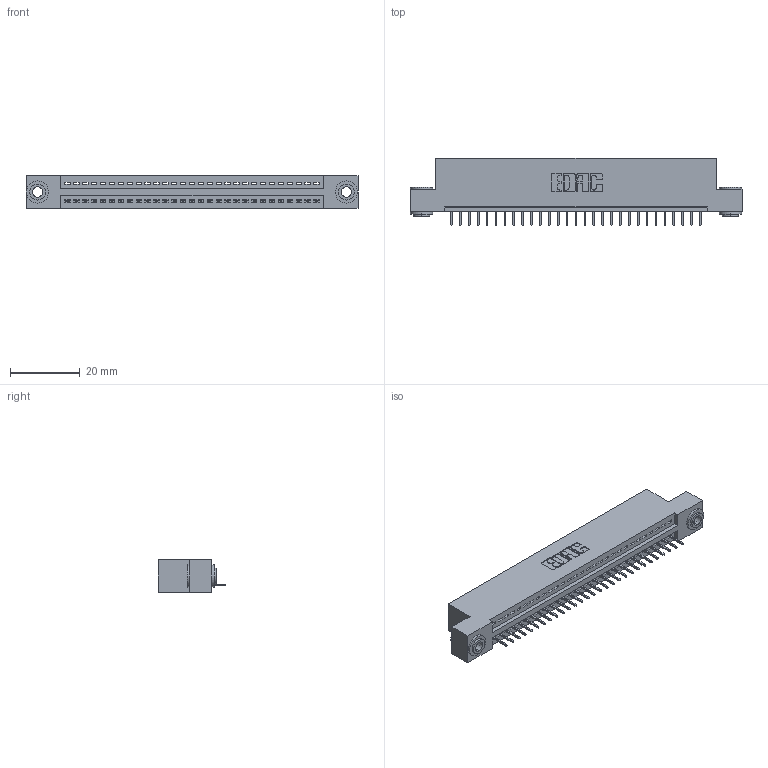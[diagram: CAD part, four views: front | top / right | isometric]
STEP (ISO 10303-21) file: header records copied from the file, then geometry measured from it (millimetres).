
FILE_DESCRIPTION (( 'STEP AP203' ), '1' );
FILE_NAME ('395-029-524-103.STEP', '2018-11-10T18:39:11', ( '' ), ( '' ), 'SwSTEP 2.0', 'SolidWorks 2016', '' );
FILE_SCHEMA (( 'CONFIG_CONTROL_DESIGN' ));
Length unit declared in the file: inch
Products named in the file (4): 395-029-524-103; 345-250-002_345-250-002-102; 345 Part_Flush Mounting Lugs - 0.156 Dia-TH; 345-292-001_345-293-124
Assembly tree (32 placements, depth 2):
  395-029-524-103
    345 Part_Flush Mounting Lugs - 0.156 Dia-TH
    345-292-001_345-293-124  x29
    345-250-002_345-250-002-102  x2
Bounding box: 94.87 x 19.35 x 9.4 mm (x, y, z)
Volume: 8809.1 mm3; surface area: 11378 mm2
Topology: 32 solids, 32 shells, 1962 faces, 5637 edges, 3638 vertices
Faces by surface type: plane 1424, cylinder 530, cone 8
Entity records: 24300 total; most frequent: CARTESIAN_POINT 4186, ORIENTED_EDGE 4142, DIRECTION 3707, EDGE_CURVE 2071, LINE 1803, VECTOR 1803, VERTEX_POINT 1374, AXIS2_PLACEMENT_3D 952
